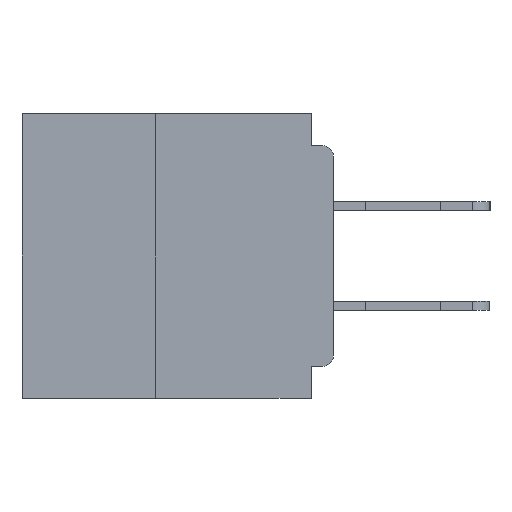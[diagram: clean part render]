
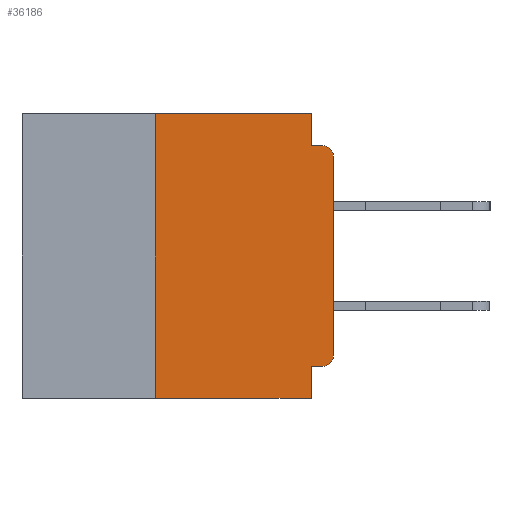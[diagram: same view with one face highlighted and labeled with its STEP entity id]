
A CAD part, left-side view. The second image highlights one B-rep face of the part: STEP entity #36186.
In plain terms, the highlighted planar face has unit normal (-1, 0, 0).
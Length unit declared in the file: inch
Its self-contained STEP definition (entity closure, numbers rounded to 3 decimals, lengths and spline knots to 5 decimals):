
#153 = CARTESIAN_POINT ( 'NONE',  ( 0., 0.031, -0.4 ) ) ;
#1435 = VERTEX_POINT ( 'NONE', #29742 ) ;
#1861 = CARTESIAN_POINT ( 'NONE',  ( 0., 0.015, -0.355 ) ) ;
#2070 = ORIENTED_EDGE ( 'NONE', *, *, #33795, .F. ) ;
#2113 = ORIENTED_EDGE ( 'NONE', *, *, #30476, .F. ) ;
#2523 = LINE ( 'NONE', #39412, #3508 ) ;
#2775 = EDGE_CURVE ( 'NONE', #25622, #1435, #31309, .T. ) ;
#3508 = VECTOR ( 'NONE', #17856, 39.37008 ) ;
#3509 = FACE_OUTER_BOUND ( 'NONE', #27055, .T. ) ;
#3851 = EDGE_CURVE ( 'NONE', #38519, #20413, #33613, .T. ) ;
#3940 = DIRECTION ( 'NONE',  ( 0., -1., 0. ) ) ;
#4349 = CARTESIAN_POINT ( 'NONE',  ( 0., 0.437, 0. ) ) ;
#4474 = DIRECTION ( 'NONE',  ( -1., 0., 0. ) ) ;
#4510 = VERTEX_POINT ( 'NONE', #13082 ) ;
#4792 = DIRECTION ( 'NONE',  ( 0., 0., 1. ) ) ;
#6149 = VECTOR ( 'NONE', #21490, 39.37008 ) ;
#7113 = ORIENTED_EDGE ( 'NONE', *, *, #3851, .F. ) ;
#8230 = AXIS2_PLACEMENT_3D ( 'NONE', #29670, #29546, #29407 ) ;
#8360 = ORIENTED_EDGE ( 'NONE', *, *, #17195, .T. ) ;
#9139 = VERTEX_POINT ( 'NONE', #1861 ) ;
#10263 = CIRCLE ( 'NONE', #33099, 0.015 ) ;
#10305 = LINE ( 'NONE', #36215, #33973 ) ;
#10430 = PLANE ( 'NONE',  #26211 ) ;
#10574 = DIRECTION ( 'NONE',  ( 1., 0., 0. ) ) ;
#11469 = LINE ( 'NONE', #22444, #27883 ) ;
#12192 = CARTESIAN_POINT ( 'NONE',  ( 0., 0., -0.045 ) ) ;
#12311 = EDGE_CURVE ( 'NONE', #15063, #30702, #2523, .T. ) ;
#12831 = VECTOR ( 'NONE', #31978, 39.37008 ) ;
#13082 = CARTESIAN_POINT ( 'NONE',  ( 0., 0., -0.34 ) ) ;
#13944 = LINE ( 'NONE', #23624, #37568 ) ;
#15063 = VERTEX_POINT ( 'NONE', #29809 ) ;
#16277 = CARTESIAN_POINT ( 'NONE',  ( 0., 0.031, -0.4 ) ) ;
#17195 = EDGE_CURVE ( 'NONE', #4510, #25622, #25405, .T. ) ;
#17689 = VERTEX_POINT ( 'NONE', #38085 ) ;
#17754 = DIRECTION ( 'NONE',  ( 0., -1., 0. ) ) ;
#17856 = DIRECTION ( 'NONE',  ( 0., 0., 1. ) ) ;
#20413 = VERTEX_POINT ( 'NONE', #16277 ) ;
#21490 = DIRECTION ( 'NONE',  ( 0., -1., 0. ) ) ;
#21824 = ORIENTED_EDGE ( 'NONE', *, *, #2775, .T. ) ;
#22444 = CARTESIAN_POINT ( 'NONE',  ( 0., 0.437, -0.4 ) ) ;
#22682 = CARTESIAN_POINT ( 'NONE',  ( 0., 0., -0.355 ) ) ;
#22997 = CARTESIAN_POINT ( 'NONE',  ( 0., 0.015, -0.34 ) ) ;
#23624 = CARTESIAN_POINT ( 'NONE',  ( 0., 0.031, 0. ) ) ;
#25405 = LINE ( 'NONE', #35686, #39857 ) ;
#25419 = VECTOR ( 'NONE', #39992, 39.37008 ) ;
#25622 = VERTEX_POINT ( 'NONE', #34732 ) ;
#25799 = EDGE_CURVE ( 'NONE', #30702, #17689, #10305, .T. ) ;
#26098 = DIRECTION ( 'NONE',  ( 0., 0., -1. ) ) ;
#26211 = AXIS2_PLACEMENT_3D ( 'NONE', #4349, #10574, #32154 ) ;
#26244 = EDGE_CURVE ( 'NONE', #9139, #4510, #10263, .T. ) ;
#26721 = DIRECTION ( 'NONE',  ( 0., 0., -1. ) ) ;
#27055 = EDGE_LOOP ( 'NONE', ( #8360, #21824, #2070, #28460, #33275, #35193, #29155, #7113, #2113, #34112 ) ) ;
#27883 = VECTOR ( 'NONE', #3940, 39.37008 ) ;
#28460 = ORIENTED_EDGE ( 'NONE', *, *, #28781, .F. ) ;
#28781 = EDGE_CURVE ( 'NONE', #17689, #29266, #13944, .T. ) ;
#29155 = ORIENTED_EDGE ( 'NONE', *, *, #34308, .T. ) ;
#29266 = VERTEX_POINT ( 'NONE', #38248 ) ;
#29407 = DIRECTION ( 'NONE',  ( 0., 0., -1. ) ) ;
#29546 = DIRECTION ( 'NONE',  ( -1., 0., 0. ) ) ;
#29670 = CARTESIAN_POINT ( 'NONE',  ( 0., 0.015, -0.06 ) ) ;
#29742 = CARTESIAN_POINT ( 'NONE',  ( 0., 0.015, -0.045 ) ) ;
#29809 = CARTESIAN_POINT ( 'NONE',  ( 0., 0.25, -0.4 ) ) ;
#30476 = EDGE_CURVE ( 'NONE', #9139, #38519, #37415, .T. ) ;
#30702 = VERTEX_POINT ( 'NONE', #36261 ) ;
#30824 = LINE ( 'NONE', #12192, #6149 ) ;
#31309 = CIRCLE ( 'NONE', #8230, 0.015 ) ;
#31978 = DIRECTION ( 'NONE',  ( 0., 1., 0. ) ) ;
#32154 = DIRECTION ( 'NONE',  ( 0., 0., -1. ) ) ;
#33099 = AXIS2_PLACEMENT_3D ( 'NONE', #22997, #4474, #26098 ) ;
#33275 = ORIENTED_EDGE ( 'NONE', *, *, #25799, .F. ) ;
#33613 = LINE ( 'NONE', #153, #25419 ) ;
#33795 = EDGE_CURVE ( 'NONE', #29266, #1435, #30824, .T. ) ;
#33973 = VECTOR ( 'NONE', #17754, 39.37008 ) ;
#34112 = ORIENTED_EDGE ( 'NONE', *, *, #26244, .T. ) ;
#34308 = EDGE_CURVE ( 'NONE', #15063, #20413, #11469, .T. ) ;
#34732 = CARTESIAN_POINT ( 'NONE',  ( 0., 0., -0.06 ) ) ;
#35193 = ORIENTED_EDGE ( 'NONE', *, *, #12311, .F. ) ;
#35686 = CARTESIAN_POINT ( 'NONE',  ( 0., 0., 0. ) ) ;
#36186 = ADVANCED_FACE ( 'NONE', ( #3509 ), #10430, .F. ) ;
#36215 = CARTESIAN_POINT ( 'NONE',  ( 0., 0.437, 0. ) ) ;
#36261 = CARTESIAN_POINT ( 'NONE',  ( 0., 0.25, 0. ) ) ;
#37415 = LINE ( 'NONE', #22682, #12831 ) ;
#37568 = VECTOR ( 'NONE', #26721, 39.37008 ) ;
#38085 = CARTESIAN_POINT ( 'NONE',  ( 0., 0.031, 0. ) ) ;
#38248 = CARTESIAN_POINT ( 'NONE',  ( 0., 0.031, -0.045 ) ) ;
#38519 = VERTEX_POINT ( 'NONE', #39836 ) ;
#39412 = CARTESIAN_POINT ( 'NONE',  ( 0., 0.25, -0.4 ) ) ;
#39836 = CARTESIAN_POINT ( 'NONE',  ( 0., 0.031, -0.355 ) ) ;
#39857 = VECTOR ( 'NONE', #4792, 39.37008 ) ;
#39992 = DIRECTION ( 'NONE',  ( 0., 0., -1. ) ) ;
